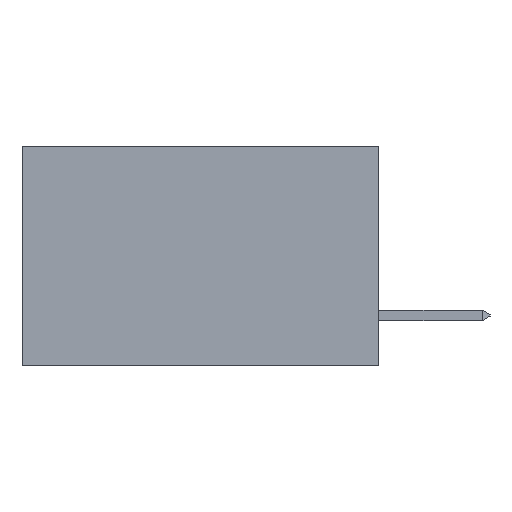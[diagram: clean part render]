
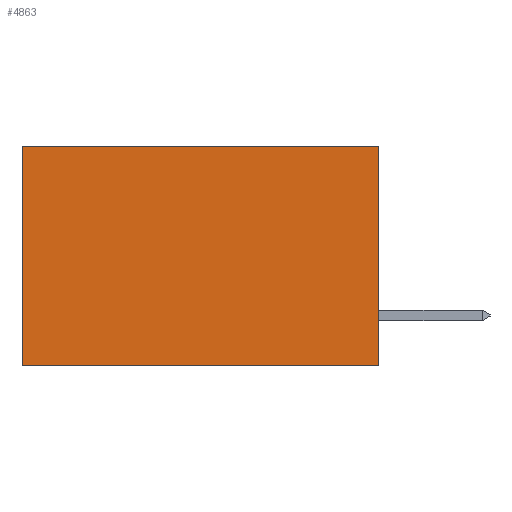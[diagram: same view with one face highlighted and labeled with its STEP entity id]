
A CAD part, left-side view. The second image highlights one B-rep face of the part: STEP entity #4863.
In plain terms, the highlighted planar face has unit normal (-1, 0, 0).
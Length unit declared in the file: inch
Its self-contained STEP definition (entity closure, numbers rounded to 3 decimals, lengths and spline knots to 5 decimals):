
#467 = VECTOR ( 'NONE', #12612, 39.37008 ) ;
#1477 = CARTESIAN_POINT ( 'NONE',  ( 0.2615, 0., 0. ) ) ;
#1637 = CARTESIAN_POINT ( 'NONE',  ( 0.2615, 0., 0. ) ) ;
#2084 = EDGE_CURVE ( 'NONE', #17972, #4938, #2363, .T. ) ;
#2363 = LINE ( 'NONE', #8355, #10416 ) ;
#2374 = LINE ( 'NONE', #4268, #17677 ) ;
#2484 = DIRECTION ( 'NONE',  ( 0., 1., 0. ) ) ;
#2725 = VERTEX_POINT ( 'NONE', #11633 ) ;
#3275 = CARTESIAN_POINT ( 'NONE',  ( 0.2615, 0.6, -0.37 ) ) ;
#4236 = DIRECTION ( 'NONE',  ( 0., 1., 0. ) ) ;
#4268 = CARTESIAN_POINT ( 'NONE',  ( 0.2615, 0., -0.37 ) ) ;
#4863 = ADVANCED_FACE ( 'NONE', ( #6074 ), #6286, .F. ) ;
#4938 = VERTEX_POINT ( 'NONE', #3275 ) ;
#5311 = ORIENTED_EDGE ( 'NONE', *, *, #10561, .F. ) ;
#5456 = EDGE_CURVE ( 'NONE', #6271, #2725, #8670, .T. ) ;
#6074 = FACE_OUTER_BOUND ( 'NONE', #18350, .T. ) ;
#6271 = VERTEX_POINT ( 'NONE', #1477 ) ;
#6286 = PLANE ( 'NONE',  #13747 ) ;
#6346 = DIRECTION ( 'NONE',  ( 0., 0., -1. ) ) ;
#6363 = DIRECTION ( 'NONE',  ( 1., 0., 0. ) ) ;
#6599 = CARTESIAN_POINT ( 'NONE',  ( 0.2615, 0., -0.37 ) ) ;
#6811 = EDGE_CURVE ( 'NONE', #6271, #17972, #15117, .T. ) ;
#7327 = CARTESIAN_POINT ( 'NONE',  ( 0.2615, 0.6, 0. ) ) ;
#7903 = DIRECTION ( 'NONE',  ( 0., 0., -1. ) ) ;
#8355 = CARTESIAN_POINT ( 'NONE',  ( 0.2615, 0.6, -0.37 ) ) ;
#8670 = LINE ( 'NONE', #12766, #467 ) ;
#10392 = ORIENTED_EDGE ( 'NONE', *, *, #2084, .T. ) ;
#10416 = VECTOR ( 'NONE', #7903, 39.37008 ) ;
#10561 = EDGE_CURVE ( 'NONE', #2725, #4938, #2374, .T. ) ;
#11633 = CARTESIAN_POINT ( 'NONE',  ( 0.2615, 0., -0.37 ) ) ;
#12612 = DIRECTION ( 'NONE',  ( 0., 0., -1. ) ) ;
#12766 = CARTESIAN_POINT ( 'NONE',  ( 0.2615, 0., -0.37 ) ) ;
#13747 = AXIS2_PLACEMENT_3D ( 'NONE', #6599, #6363, #6346 ) ;
#14409 = ORIENTED_EDGE ( 'NONE', *, *, #6811, .T. ) ;
#15117 = LINE ( 'NONE', #1637, #19020 ) ;
#17677 = VECTOR ( 'NONE', #4236, 39.37008 ) ;
#17972 = VERTEX_POINT ( 'NONE', #7327 ) ;
#18350 = EDGE_LOOP ( 'NONE', ( #10392, #5311, #18848, #14409 ) ) ;
#18848 = ORIENTED_EDGE ( 'NONE', *, *, #5456, .F. ) ;
#19020 = VECTOR ( 'NONE', #2484, 39.37008 ) ;
